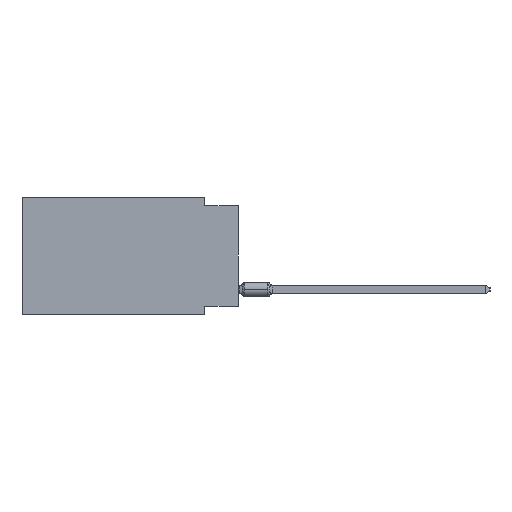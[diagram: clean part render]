
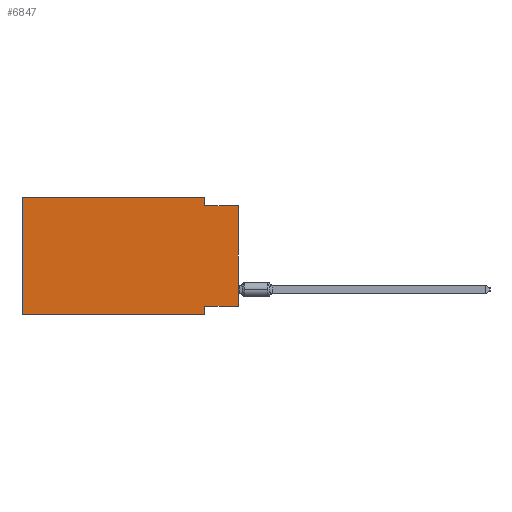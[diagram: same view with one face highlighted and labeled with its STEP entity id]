
A CAD part, left-side view. The second image highlights one B-rep face of the part: STEP entity #6847.
In plain terms, the highlighted planar face has unit normal (-1, 0, 0).
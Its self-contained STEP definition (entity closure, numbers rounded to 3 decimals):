
#27 = DIRECTION ( 'NONE',  ( 1., 0., 0. ) ) ;
#244 = LINE ( 'NONE', #68610, #60905 ) ;
#2545 = EDGE_CURVE ( 'NONE', #43151, #35420, #77479, .T. ) ;
#4716 = EDGE_CURVE ( 'NONE', #34805, #49253, #244, .T. ) ;
#4791 = CARTESIAN_POINT ( 'NONE',  ( 0., 2.54, 0. ) ) ;
#6847 = ADVANCED_FACE ( 'NONE', ( #37116 ), #16092, .F. ) ;
#7125 = VECTOR ( 'NONE', #75482, 1000. ) ;
#11373 = CARTESIAN_POINT ( 'NONE',  ( 0., 2.54, -8.89 ) ) ;
#11811 = CARTESIAN_POINT ( 'NONE',  ( 0., 0., -0.635 ) ) ;
#12954 = DIRECTION ( 'NONE',  ( 0., 0., 1. ) ) ;
#14541 = EDGE_CURVE ( 'NONE', #19230, #49253, #70168, .T. ) ;
#16036 = LINE ( 'NONE', #39446, #72251 ) ;
#16092 = PLANE ( 'NONE',  #48660 ) ;
#16116 = EDGE_LOOP ( 'NONE', ( #17100, #56140, #94571, #67467, #36769, #29127, #86364, #41727 ) ) ;
#17100 = ORIENTED_EDGE ( 'NONE', *, *, #14541, .T. ) ;
#17362 = CARTESIAN_POINT ( 'NONE',  ( 0., 0., -8.255 ) ) ;
#19230 = VERTEX_POINT ( 'NONE', #17362 ) ;
#21175 = DIRECTION ( 'NONE',  ( 0., 1., 0. ) ) ;
#23159 = CARTESIAN_POINT ( 'NONE',  ( 0., 2.54, -0.635 ) ) ;
#23494 = EDGE_CURVE ( 'NONE', #78805, #42495, #86134, .T. ) ;
#23864 = CARTESIAN_POINT ( 'NONE',  ( 0., 2.54, -8.89 ) ) ;
#27518 = LINE ( 'NONE', #42688, #37034 ) ;
#29127 = ORIENTED_EDGE ( 'NONE', *, *, #88743, .T. ) ;
#30362 = EDGE_CURVE ( 'NONE', #35420, #34805, #16036, .T. ) ;
#31644 = DIRECTION ( 'NONE',  ( 0., 0., -1. ) ) ;
#34805 = VERTEX_POINT ( 'NONE', #23159 ) ;
#35420 = VERTEX_POINT ( 'NONE', #4791 ) ;
#36769 = ORIENTED_EDGE ( 'NONE', *, *, #58032, .F. ) ;
#37034 = VECTOR ( 'NONE', #21175, 1000. ) ;
#37116 = FACE_OUTER_BOUND ( 'NONE', #16116, .T. ) ;
#39446 = CARTESIAN_POINT ( 'NONE',  ( 0., 2.54, 0. ) ) ;
#39727 = DIRECTION ( 'NONE',  ( 0., 0., -1. ) ) ;
#40334 = DIRECTION ( 'NONE',  ( 0., -1., 0. ) ) ;
#40945 = CARTESIAN_POINT ( 'NONE',  ( 0., 16.383, 0. ) ) ;
#41727 = ORIENTED_EDGE ( 'NONE', *, *, #59908, .F. ) ;
#42495 = VERTEX_POINT ( 'NONE', #23864 ) ;
#42688 = CARTESIAN_POINT ( 'NONE',  ( 0., 0., -8.255 ) ) ;
#43151 = VERTEX_POINT ( 'NONE', #88683 ) ;
#47192 = CARTESIAN_POINT ( 'NONE',  ( 0., 16.383, 0. ) ) ;
#48660 = AXIS2_PLACEMENT_3D ( 'NONE', #66946, #27, #52287 ) ;
#49253 = VERTEX_POINT ( 'NONE', #11811 ) ;
#52287 = DIRECTION ( 'NONE',  ( 0., 0., -1. ) ) ;
#56103 = DIRECTION ( 'NONE',  ( 0., 0., 1. ) ) ;
#56125 = VERTEX_POINT ( 'NONE', #86607 ) ;
#56140 = ORIENTED_EDGE ( 'NONE', *, *, #4716, .F. ) ;
#58032 = EDGE_CURVE ( 'NONE', #56125, #43151, #85435, .T. ) ;
#59908 = EDGE_CURVE ( 'NONE', #19230, #78805, #27518, .T. ) ;
#60905 = VECTOR ( 'NONE', #82801, 1000. ) ;
#66946 = CARTESIAN_POINT ( 'NONE',  ( 0., 16.383, 0. ) ) ;
#67467 = ORIENTED_EDGE ( 'NONE', *, *, #2545, .F. ) ;
#67677 = VECTOR ( 'NONE', #39727, 1000. ) ;
#68610 = CARTESIAN_POINT ( 'NONE',  ( 0., 0., -0.635 ) ) ;
#70168 = LINE ( 'NONE', #79904, #83561 ) ;
#72251 = VECTOR ( 'NONE', #31644, 1000. ) ;
#75482 = DIRECTION ( 'NONE',  ( 0., -1., 0. ) ) ;
#77479 = LINE ( 'NONE', #47192, #94934 ) ;
#78805 = VERTEX_POINT ( 'NONE', #91709 ) ;
#79904 = CARTESIAN_POINT ( 'NONE',  ( 0., 0., 0. ) ) ;
#80904 = LINE ( 'NONE', #82832, #7125 ) ;
#82801 = DIRECTION ( 'NONE',  ( 0., -1., 0. ) ) ;
#82832 = CARTESIAN_POINT ( 'NONE',  ( 0., 16.383, -8.89 ) ) ;
#83561 = VECTOR ( 'NONE', #12954, 1000. ) ;
#85435 = LINE ( 'NONE', #40945, #96148 ) ;
#86134 = LINE ( 'NONE', #11373, #67677 ) ;
#86364 = ORIENTED_EDGE ( 'NONE', *, *, #23494, .F. ) ;
#86607 = CARTESIAN_POINT ( 'NONE',  ( 0., 16.383, -8.89 ) ) ;
#88683 = CARTESIAN_POINT ( 'NONE',  ( 0., 16.383, 0. ) ) ;
#88743 = EDGE_CURVE ( 'NONE', #56125, #42495, #80904, .T. ) ;
#91709 = CARTESIAN_POINT ( 'NONE',  ( 0., 2.54, -8.255 ) ) ;
#94571 = ORIENTED_EDGE ( 'NONE', *, *, #30362, .F. ) ;
#94934 = VECTOR ( 'NONE', #40334, 1000. ) ;
#96148 = VECTOR ( 'NONE', #56103, 1000. ) ;
